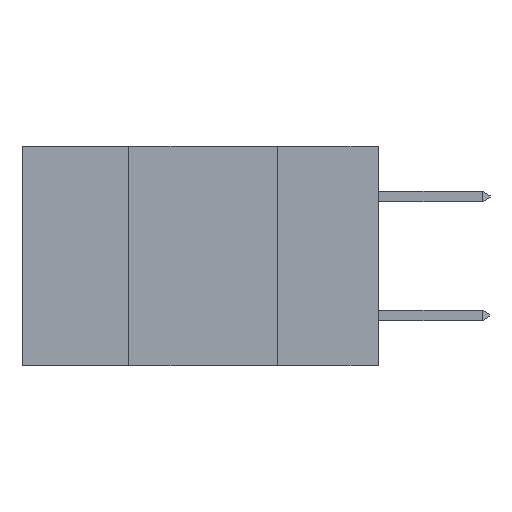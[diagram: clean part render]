
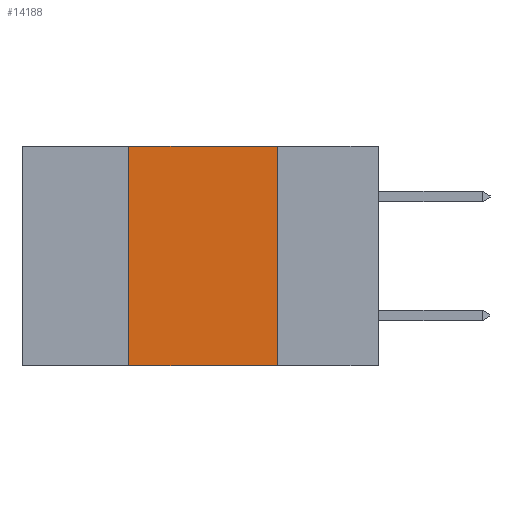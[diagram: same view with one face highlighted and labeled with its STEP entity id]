
A CAD part, left-side view. The second image highlights one B-rep face of the part: STEP entity #14188.
In plain terms, the highlighted planar face has unit normal (-1, 0, 0).
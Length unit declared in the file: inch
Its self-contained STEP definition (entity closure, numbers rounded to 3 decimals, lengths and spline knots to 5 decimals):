
#74 = DIRECTION ( 'NONE',  ( 0., -1., 0. ) ) ;
#220 = CARTESIAN_POINT ( 'NONE',  ( 0., 0.17, -0.37 ) ) ;
#664 = ORIENTED_EDGE ( 'NONE', *, *, #22082, .F. ) ;
#1900 = ORIENTED_EDGE ( 'NONE', *, *, #7481, .F. ) ;
#2011 = VERTEX_POINT ( 'NONE', #6296 ) ;
#2070 = LINE ( 'NONE', #22193, #15779 ) ;
#2988 = FACE_OUTER_BOUND ( 'NONE', #15570, .T. ) ;
#4662 = VERTEX_POINT ( 'NONE', #17953 ) ;
#4839 = ORIENTED_EDGE ( 'NONE', *, *, #10418, .F. ) ;
#4936 = CARTESIAN_POINT ( 'NONE',  ( 0., 0.17, -0.37 ) ) ;
#5101 = DIRECTION ( 'NONE',  ( 1., 0., 0. ) ) ;
#6113 = VECTOR ( 'NONE', #9756, 39.37008 ) ;
#6296 = CARTESIAN_POINT ( 'NONE',  ( 0., 0.42, 0. ) ) ;
#7481 = EDGE_CURVE ( 'NONE', #18330, #2011, #9538, .T. ) ;
#7878 = CARTESIAN_POINT ( 'NONE',  ( 0., 0.6, -0.37 ) ) ;
#8697 = CARTESIAN_POINT ( 'NONE',  ( 0., 0.42, -0.37 ) ) ;
#9538 = LINE ( 'NONE', #10630, #13857 ) ;
#9756 = DIRECTION ( 'NONE',  ( 0., -1., 0. ) ) ;
#10418 = EDGE_CURVE ( 'NONE', #4662, #19903, #22152, .T. ) ;
#10630 = CARTESIAN_POINT ( 'NONE',  ( 0., 0.42, -0.37 ) ) ;
#10661 = CARTESIAN_POINT ( 'NONE',  ( 0., 0.6, 0. ) ) ;
#12460 = DIRECTION ( 'NONE',  ( 0., 0., -1. ) ) ;
#13857 = VECTOR ( 'NONE', #17942, 39.37008 ) ;
#14188 = ADVANCED_FACE ( 'NONE', ( #2988 ), #16184, .F. ) ;
#15570 = EDGE_LOOP ( 'NONE', ( #4839, #664, #1900, #21183 ) ) ;
#15779 = VECTOR ( 'NONE', #74, 39.37008 ) ;
#16184 = PLANE ( 'NONE',  #19805 ) ;
#17404 = VECTOR ( 'NONE', #12460, 39.37008 ) ;
#17942 = DIRECTION ( 'NONE',  ( 0., 0., 1. ) ) ;
#17953 = CARTESIAN_POINT ( 'NONE',  ( 0., 0.17, 0. ) ) ;
#17971 = DIRECTION ( 'NONE',  ( 0., 0., -1. ) ) ;
#18330 = VERTEX_POINT ( 'NONE', #8697 ) ;
#19805 = AXIS2_PLACEMENT_3D ( 'NONE', #10661, #5101, #17971 ) ;
#19903 = VERTEX_POINT ( 'NONE', #220 ) ;
#20667 = LINE ( 'NONE', #7878, #6113 ) ;
#21183 = ORIENTED_EDGE ( 'NONE', *, *, #22805, .T. ) ;
#22082 = EDGE_CURVE ( 'NONE', #2011, #4662, #2070, .T. ) ;
#22152 = LINE ( 'NONE', #4936, #17404 ) ;
#22193 = CARTESIAN_POINT ( 'NONE',  ( 0., 0.6, 0. ) ) ;
#22805 = EDGE_CURVE ( 'NONE', #18330, #19903, #20667, .T. ) ;
